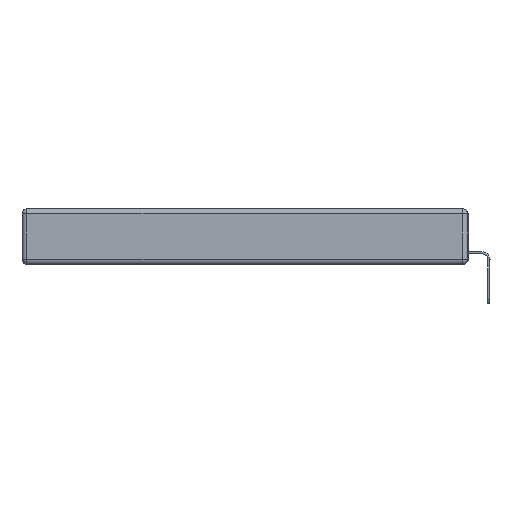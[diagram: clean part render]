
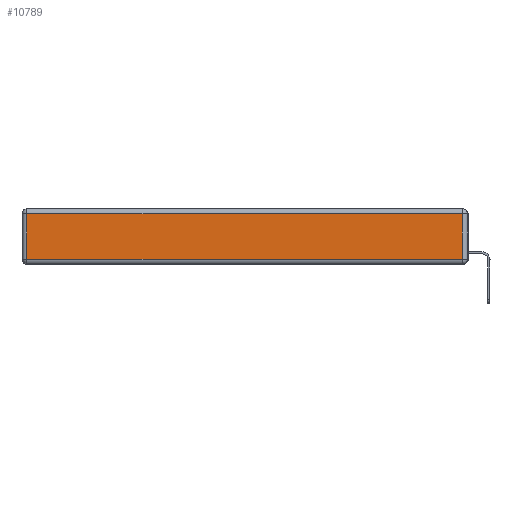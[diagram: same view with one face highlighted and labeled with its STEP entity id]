
A CAD part, left-side view. The second image highlights one B-rep face of the part: STEP entity #10789.
In plain terms, the highlighted planar face has unit normal (-1, 0, 0).
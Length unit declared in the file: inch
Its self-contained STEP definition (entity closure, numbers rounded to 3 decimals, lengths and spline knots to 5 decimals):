
#287 = CARTESIAN_POINT ( 'NONE',  ( 0., 0.03, -0.343 ) ) ;
#828 = VECTOR ( 'NONE', #15341, 39.37008 ) ;
#1375 = EDGE_LOOP ( 'NONE', ( #9822, #15692, #10535, #11609 ) ) ;
#1448 = PLANE ( 'NONE',  #14042 ) ;
#1528 = DIRECTION ( 'NONE',  ( 0., 0., 1. ) ) ;
#2741 = CARTESIAN_POINT ( 'NONE',  ( 0., 0.03, -0.313 ) ) ;
#3355 = CARTESIAN_POINT ( 'NONE',  ( 0., 2.72, -0.313 ) ) ;
#3376 = LINE ( 'NONE', #5349, #828 ) ;
#4566 = EDGE_CURVE ( 'NONE', #6644, #12671, #11482, .T. ) ;
#5158 = CARTESIAN_POINT ( 'NONE',  ( 0., 0., -0.343 ) ) ;
#5349 = CARTESIAN_POINT ( 'NONE',  ( 0., 2.72, -0.343 ) ) ;
#5637 = VECTOR ( 'NONE', #16101, 39.37008 ) ;
#6139 = CARTESIAN_POINT ( 'NONE',  ( 0., 0., -0.313 ) ) ;
#6644 = VERTEX_POINT ( 'NONE', #3355 ) ;
#8848 = CARTESIAN_POINT ( 'NONE',  ( 0., 2.72, -0.03 ) ) ;
#8996 = DIRECTION ( 'NONE',  ( 0., 0., 1. ) ) ;
#9241 = LINE ( 'NONE', #12352, #12164 ) ;
#9415 = VECTOR ( 'NONE', #1528, 39.37008 ) ;
#9537 = FACE_OUTER_BOUND ( 'NONE', #1375, .T. ) ;
#9779 = EDGE_CURVE ( 'NONE', #12767, #6644, #3376, .T. ) ;
#9822 = ORIENTED_EDGE ( 'NONE', *, *, #4566, .T. ) ;
#10144 = CARTESIAN_POINT ( 'NONE',  ( 0., 0.03, -0.03 ) ) ;
#10535 = ORIENTED_EDGE ( 'NONE', *, *, #13872, .T. ) ;
#10789 = ADVANCED_FACE ( 'NONE', ( #9537 ), #1448, .T. ) ;
#11451 = DIRECTION ( 'NONE',  ( -1., 0., 0. ) ) ;
#11482 = LINE ( 'NONE', #6139, #5637 ) ;
#11609 = ORIENTED_EDGE ( 'NONE', *, *, #9779, .T. ) ;
#12164 = VECTOR ( 'NONE', #15954, 39.37008 ) ;
#12352 = CARTESIAN_POINT ( 'NONE',  ( 0., 2.75, -0.03 ) ) ;
#12671 = VERTEX_POINT ( 'NONE', #2741 ) ;
#12767 = VERTEX_POINT ( 'NONE', #8848 ) ;
#13872 = EDGE_CURVE ( 'NONE', #15633, #12767, #9241, .T. ) ;
#14042 = AXIS2_PLACEMENT_3D ( 'NONE', #5158, #11451, #8996 ) ;
#14220 = EDGE_CURVE ( 'NONE', #12671, #15633, #16065, .T. ) ;
#15341 = DIRECTION ( 'NONE',  ( 0., 0., -1. ) ) ;
#15633 = VERTEX_POINT ( 'NONE', #10144 ) ;
#15692 = ORIENTED_EDGE ( 'NONE', *, *, #14220, .T. ) ;
#15954 = DIRECTION ( 'NONE',  ( 0., 1., 0. ) ) ;
#16065 = LINE ( 'NONE', #287, #9415 ) ;
#16101 = DIRECTION ( 'NONE',  ( 0., -1., 0. ) ) ;
